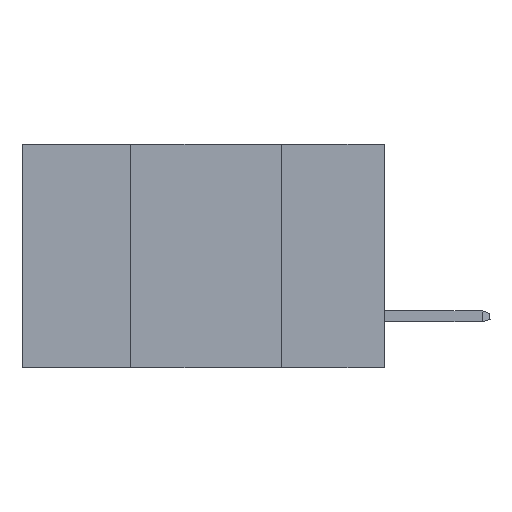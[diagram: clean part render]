
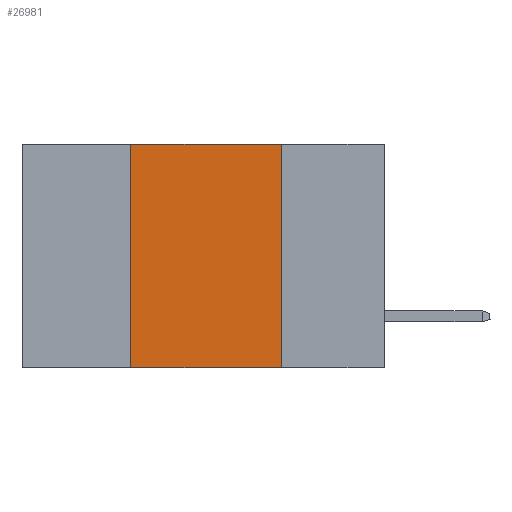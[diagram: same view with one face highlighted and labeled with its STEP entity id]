
A CAD part, left-side view. The second image highlights one B-rep face of the part: STEP entity #26981.
In plain terms, the highlighted planar face has unit normal (-1, 0, 0).
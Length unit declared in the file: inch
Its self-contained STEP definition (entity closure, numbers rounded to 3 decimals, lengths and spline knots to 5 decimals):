
#3 = CARTESIAN_POINT ( 'NONE',  ( 0., 0.42, 0. ) ) ;
#198 = ORIENTED_EDGE ( 'NONE', *, *, #4894, .F. ) ;
#1411 = ORIENTED_EDGE ( 'NONE', *, *, #27354, .F. ) ;
#2306 = VERTEX_POINT ( 'NONE', #18944 ) ;
#3340 = VERTEX_POINT ( 'NONE', #20918 ) ;
#3610 = ORIENTED_EDGE ( 'NONE', *, *, #14038, .F. ) ;
#3837 = CARTESIAN_POINT ( 'NONE',  ( 0., 0.42, 0. ) ) ;
#4894 = EDGE_CURVE ( 'NONE', #15995, #17119, #7726, .T. ) ;
#5035 = CARTESIAN_POINT ( 'NONE',  ( 0., 0.6, -0.37 ) ) ;
#6164 = CARTESIAN_POINT ( 'NONE',  ( 0., 0.17, 0. ) ) ;
#6921 = CARTESIAN_POINT ( 'NONE',  ( 0., 0.17, 0. ) ) ;
#7726 = LINE ( 'NONE', #19201, #12910 ) ;
#7855 = LINE ( 'NONE', #5035, #16438 ) ;
#7998 = DIRECTION ( 'NONE',  ( 0., 0., -1. ) ) ;
#9715 = LINE ( 'NONE', #6164, #10055 ) ;
#9800 = PLANE ( 'NONE',  #14802 ) ;
#9848 = ORIENTED_EDGE ( 'NONE', *, *, #18701, .T. ) ;
#10055 = VECTOR ( 'NONE', #26075, 39.37008 ) ;
#10286 = EDGE_LOOP ( 'NONE', ( #1411, #198, #3610, #9848 ) ) ;
#12910 = VECTOR ( 'NONE', #17233, 39.37008 ) ;
#13642 = DIRECTION ( 'NONE',  ( 0., 0., 1. ) ) ;
#14038 = EDGE_CURVE ( 'NONE', #2306, #15995, #19115, .T. ) ;
#14432 = DIRECTION ( 'NONE',  ( 1., 0., 0. ) ) ;
#14802 = AXIS2_PLACEMENT_3D ( 'NONE', #18887, #14432, #7998 ) ;
#15608 = FACE_OUTER_BOUND ( 'NONE', #10286, .T. ) ;
#15995 = VERTEX_POINT ( 'NONE', #3837 ) ;
#16438 = VECTOR ( 'NONE', #20315, 39.37008 ) ;
#17119 = VERTEX_POINT ( 'NONE', #6921 ) ;
#17233 = DIRECTION ( 'NONE',  ( 0., -1., 0. ) ) ;
#18701 = EDGE_CURVE ( 'NONE', #2306, #3340, #7855, .T. ) ;
#18887 = CARTESIAN_POINT ( 'NONE',  ( 0., 0.6, 0. ) ) ;
#18944 = CARTESIAN_POINT ( 'NONE',  ( 0., 0.42, -0.37 ) ) ;
#19115 = LINE ( 'NONE', #3, #28074 ) ;
#19201 = CARTESIAN_POINT ( 'NONE',  ( 0., 0.6, 0. ) ) ;
#20315 = DIRECTION ( 'NONE',  ( 0., -1., 0. ) ) ;
#20918 = CARTESIAN_POINT ( 'NONE',  ( 0., 0.17, -0.37 ) ) ;
#26075 = DIRECTION ( 'NONE',  ( 0., 0., -1. ) ) ;
#26981 = ADVANCED_FACE ( 'NONE', ( #15608 ), #9800, .F. ) ;
#27354 = EDGE_CURVE ( 'NONE', #17119, #3340, #9715, .T. ) ;
#28074 = VECTOR ( 'NONE', #13642, 39.37008 ) ;
